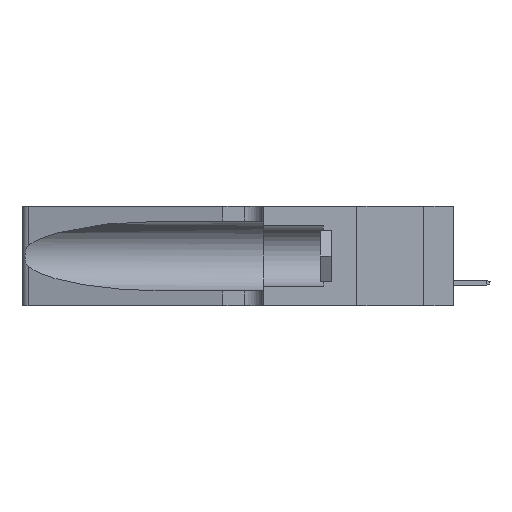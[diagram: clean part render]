
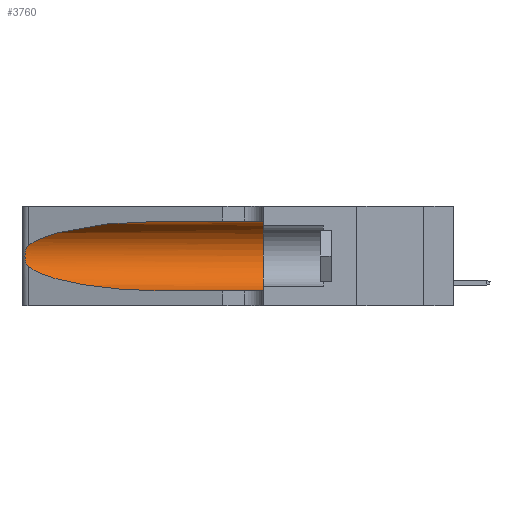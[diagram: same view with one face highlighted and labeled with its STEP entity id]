
A CAD part, left-side view. The second image highlights one B-rep face of the part: STEP entity #3760.
In plain terms, the highlighted cylindrical face has radius 3.308 mm (diameter 6.617 mm), a partial arc.
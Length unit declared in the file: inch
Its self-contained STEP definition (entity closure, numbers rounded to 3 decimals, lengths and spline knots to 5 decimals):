
#19 = DIRECTION ( 'NONE',  ( 0., 0., 1. ) ) ;
#253 = CARTESIAN_POINT ( 'NONE',  ( 0.26075, 1.23896, 0.178 ) ) ;
#1334 =( BOUNDED_CURVE ( )  B_SPLINE_CURVE ( 3, ( #7270, #7427, #21131, #18287 ),
 .UNSPECIFIED., .F., .T. ) 
 B_SPLINE_CURVE_WITH_KNOTS ( ( 4, 4 ),
 ( 3.44316, 4.71239 ),
 .UNSPECIFIED. ) 
 CURVE ( )  GEOMETRIC_REPRESENTATION_ITEM ( )  RATIONAL_B_SPLINE_CURVE ( ( 1., 0.87, 0.87, 1. ) ) 
 REPRESENTATION_ITEM ( '' )  );
#1891 = VERTEX_POINT ( 'NONE', #35018 ) ;
#2915 = VERTEX_POINT ( 'NONE', #24876 ) ;
#2934 = CARTESIAN_POINT ( 'NONE',  ( 0.25854, 1.2359, 0.20912 ) ) ;
#3012 = DIRECTION ( 'NONE',  ( 0., -1., 0. ) ) ;
#3221 = VECTOR ( 'NONE', #31213, 39.37008 ) ;
#3579 =( BOUNDED_CURVE ( )  B_SPLINE_CURVE ( 3, ( #4379, #15241, #12037, #26095 ),
 .UNSPECIFIED., .F., .T. ) 
 B_SPLINE_CURVE_WITH_KNOTS ( ( 4, 4 ),
 ( 1.5708, 2.84003 ),
 .UNSPECIFIED. ) 
 CURVE ( )  GEOMETRIC_REPRESENTATION_ITEM ( )  RATIONAL_B_SPLINE_CURVE ( ( 1., 0.87, 0.87, 1. ) ) 
 REPRESENTATION_ITEM ( '' )  );
#3718 = CYLINDRICAL_SURFACE ( 'NONE', #23966, 0.13025 ) ;
#3760 = ADVANCED_FACE ( 'NONE', ( #17229 ), #3718, .F. ) ;
#4379 = CARTESIAN_POINT ( 'NONE',  ( 0.1305, 0.72297, 0.31525 ) ) ;
#4720 = LINE ( 'NONE', #33963, #25525 ) ;
#5420 = CARTESIAN_POINT ( 'NONE',  ( 0.25487, 1.22718, 0.22369 ) ) ;
#7270 = CARTESIAN_POINT ( 'NONE',  ( 0.25487, 1.22718, 0.14631 ) ) ;
#7427 = CARTESIAN_POINT ( 'NONE',  ( 0.2373, 1.15595, 0.08982 ) ) ;
#7855 = DIRECTION ( 'NONE',  ( 0., 1., 0. ) ) ;
#8426 = CARTESIAN_POINT ( 'NONE',  ( 0.25789, 1.23486, 0.15765 ) ) ;
#9078 = CARTESIAN_POINT ( 'NONE',  ( 0.1305, 0.72297, 0.31525 ) ) ;
#9517 = ORIENTED_EDGE ( 'NONE', *, *, #12855, .F. ) ;
#9528 = DIRECTION ( 'NONE',  ( 0., -1., 0. ) ) ;
#10035 = EDGE_CURVE ( 'NONE', #2915, #34700, #1334, .T. ) ;
#10062 = CARTESIAN_POINT ( 'NONE',  ( 0.1305, 0.72297, 0.05475 ) ) ;
#10879 = CARTESIAN_POINT ( 'NONE',  ( 0.1305, 0.35, 0.185 ) ) ;
#11457 = CARTESIAN_POINT ( 'NONE',  ( 0.25639, 1.23186, 0.15144 ) ) ;
#11964 = EDGE_LOOP ( 'NONE', ( #28497, #33281, #32802, #18886, #12187, #9517 ) ) ;
#12037 = CARTESIAN_POINT ( 'NONE',  ( 0.2373, 1.15595, 0.28018 ) ) ;
#12187 = ORIENTED_EDGE ( 'NONE', *, *, #32276, .F. ) ;
#12326 = CARTESIAN_POINT ( 'NONE',  ( 0.25487, 1.22718, 0.22369 ) ) ;
#12437 = VERTEX_POINT ( 'NONE', #32031 ) ;
#12855 = EDGE_CURVE ( 'NONE', #17559, #1891, #4720, .T. ) ;
#13772 = CARTESIAN_POINT ( 'NONE',  ( 0.26018, 1.23835, 0.19895 ) ) ;
#15241 = CARTESIAN_POINT ( 'NONE',  ( 0.18966, 0.96281, 0.31525 ) ) ;
#15502 = CARTESIAN_POINT ( 'NONE',  ( 0.1305, 1.61858, 0.05475 ) ) ;
#15688 = LINE ( 'NONE', #15502, #3221 ) ;
#16296 = CARTESIAN_POINT ( 'NONE',  ( 0.25555, 1.22994, 0.2215 ) ) ;
#16531 = CARTESIAN_POINT ( 'NONE',  ( 0.1305, 1.61858, 0.185 ) ) ;
#17208 = AXIS2_PLACEMENT_3D ( 'NONE', #10879, #7855, #19 ) ;
#17229 = FACE_OUTER_BOUND ( 'NONE', #11964, .T. ) ;
#17559 = VERTEX_POINT ( 'NONE', #9078 ) ;
#18287 = CARTESIAN_POINT ( 'NONE',  ( 0.1305, 0.72297, 0.05475 ) ) ;
#18886 = ORIENTED_EDGE ( 'NONE', *, *, #24908, .T. ) ;
#19817 = CARTESIAN_POINT ( 'NONE',  ( 0.25487, 1.22718, 0.14631 ) ) ;
#20688 = B_SPLINE_CURVE_WITH_KNOTS ( 'NONE', 3,
 ( #5420, #16296, #27335, #24836, #2934, #13772, #24656, #253, #21987, #32866, #8426, #11457, #22331, #19817 ),
 .UNSPECIFIED., .F., .F.,
 ( 4, 2, 2, 2, 2, 2, 4 ),
 ( 0., 0.00027, 0.00053, 0.00107, 0.0016, 0.00187, 0.00214 ),
 .UNSPECIFIED. ) ;
#21131 = CARTESIAN_POINT ( 'NONE',  ( 0.18966, 0.96281, 0.05475 ) ) ;
#21987 = CARTESIAN_POINT ( 'NONE',  ( 0.26017, 1.23833, 0.17102 ) ) ;
#22331 = CARTESIAN_POINT ( 'NONE',  ( 0.25555, 1.22993, 0.14849 ) ) ;
#23838 = EDGE_CURVE ( 'NONE', #26156, #2915, #20688, .T. ) ;
#23966 = AXIS2_PLACEMENT_3D ( 'NONE', #16531, #3012, #27409 ) ;
#24656 = CARTESIAN_POINT ( 'NONE',  ( 0.26075, 1.23896, 0.19203 ) ) ;
#24836 = CARTESIAN_POINT ( 'NONE',  ( 0.25787, 1.23484, 0.2124 ) ) ;
#24876 = CARTESIAN_POINT ( 'NONE',  ( 0.25487, 1.22718, 0.14631 ) ) ;
#24908 = EDGE_CURVE ( 'NONE', #34700, #12437, #15688, .T. ) ;
#25180 = CIRCLE ( 'NONE', #17208, 0.13025 ) ;
#25525 = VECTOR ( 'NONE', #9528, 39.37008 ) ;
#26095 = CARTESIAN_POINT ( 'NONE',  ( 0.25487, 1.22718, 0.22369 ) ) ;
#26156 = VERTEX_POINT ( 'NONE', #12326 ) ;
#27335 = CARTESIAN_POINT ( 'NONE',  ( 0.25639, 1.23184, 0.21858 ) ) ;
#27409 = DIRECTION ( 'NONE',  ( 0., 0., -1. ) ) ;
#28497 = ORIENTED_EDGE ( 'NONE', *, *, #34673, .T. ) ;
#31213 = DIRECTION ( 'NONE',  ( 0., -1., 0. ) ) ;
#32031 = CARTESIAN_POINT ( 'NONE',  ( 0.1305, 0.35, 0.05475 ) ) ;
#32276 = EDGE_CURVE ( 'NONE', #1891, #12437, #25180, .T. ) ;
#32802 = ORIENTED_EDGE ( 'NONE', *, *, #10035, .T. ) ;
#32866 = CARTESIAN_POINT ( 'NONE',  ( 0.25856, 1.23593, 0.16098 ) ) ;
#33281 = ORIENTED_EDGE ( 'NONE', *, *, #23838, .T. ) ;
#33963 = CARTESIAN_POINT ( 'NONE',  ( 0.1305, 1.61858, 0.31525 ) ) ;
#34673 = EDGE_CURVE ( 'NONE', #17559, #26156, #3579, .T. ) ;
#34700 = VERTEX_POINT ( 'NONE', #10062 ) ;
#35018 = CARTESIAN_POINT ( 'NONE',  ( 0.1305, 0.35, 0.31525 ) ) ;
